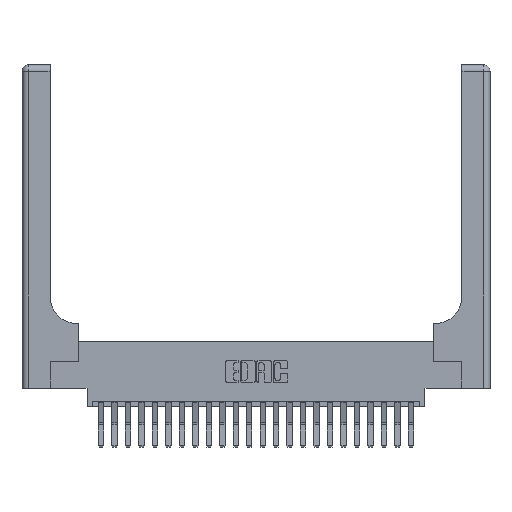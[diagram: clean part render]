
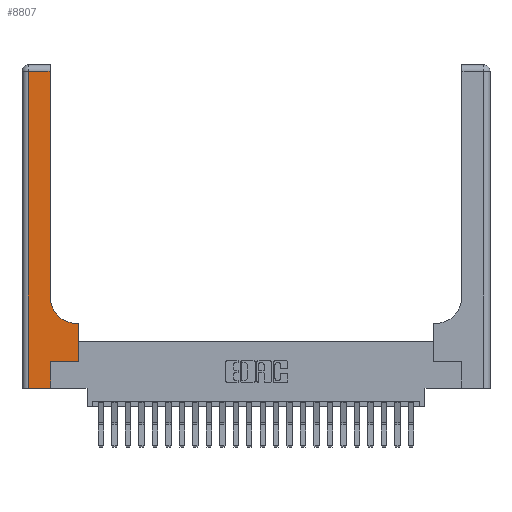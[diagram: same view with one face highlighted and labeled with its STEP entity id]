
A CAD part, top view. The second image highlights one B-rep face of the part: STEP entity #8807.
In plain terms, the highlighted planar face has unit normal (0, 0, 1).
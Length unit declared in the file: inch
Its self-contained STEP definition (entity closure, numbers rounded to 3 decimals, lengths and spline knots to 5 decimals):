
#568 = CARTESIAN_POINT ( 'NONE',  ( 0.265, 0., 0.37 ) ) ;
#609 = LINE ( 'NONE', #568, #10278 ) ;
#638 = CARTESIAN_POINT ( 'NONE',  ( 0.265, 0.25, 0.37 ) ) ;
#808 = ORIENTED_EDGE ( 'NONE', *, *, #5262, .T. ) ;
#1343 = CARTESIAN_POINT ( 'NONE',  ( 0.26, 0.6, 0.37 ) ) ;
#1937 = VERTEX_POINT ( 'NONE', #22433 ) ;
#2376 = ORIENTED_EDGE ( 'NONE', *, *, #13776, .T. ) ;
#2564 = AXIS2_PLACEMENT_3D ( 'NONE', #23322, #5184, #17915 ) ;
#2583 = DIRECTION ( 'NONE',  ( 0., 1., 0. ) ) ;
#2794 = CARTESIAN_POINT ( 'NONE',  ( 0.265, 0., 0.37 ) ) ;
#3011 = CARTESIAN_POINT ( 'NONE',  ( 0.26, 0.85, 0.37 ) ) ;
#3311 = FACE_OUTER_BOUND ( 'NONE', #10077, .T. ) ;
#4153 = EDGE_CURVE ( 'NONE', #20471, #22160, #22026, .T. ) ;
#4465 = VERTEX_POINT ( 'NONE', #6949 ) ;
#5184 = DIRECTION ( 'NONE',  ( 0., 0., -1. ) ) ;
#5262 = EDGE_CURVE ( 'NONE', #18649, #18373, #609, .T. ) ;
#5663 = LINE ( 'NONE', #18092, #20139 ) ;
#5691 = CARTESIAN_POINT ( 'NONE',  ( 0.51, 0.85, 0.37 ) ) ;
#5814 = EDGE_CURVE ( 'NONE', #19617, #18649, #13933, .T. ) ;
#6398 = ORIENTED_EDGE ( 'NONE', *, *, #19377, .T. ) ;
#6949 = CARTESIAN_POINT ( 'NONE',  ( 0.26, 2.94, 0.37 ) ) ;
#7015 = CARTESIAN_POINT ( 'NONE',  ( 0., 0., 0.37 ) ) ;
#7230 = ORIENTED_EDGE ( 'NONE', *, *, #4153, .T. ) ;
#7410 = CARTESIAN_POINT ( 'NONE',  ( 0.06, 0., 0.37 ) ) ;
#7495 = DIRECTION ( 'NONE',  ( 1., 0., 0. ) ) ;
#8097 = CARTESIAN_POINT ( 'NONE',  ( 0.528, 0.6, 0.37 ) ) ;
#8179 = VERTEX_POINT ( 'NONE', #3011 ) ;
#8243 = VECTOR ( 'NONE', #8671, 39.37008 ) ;
#8302 = EDGE_CURVE ( 'NONE', #21904, #8179, #17270, .T. ) ;
#8671 = DIRECTION ( 'NONE',  ( 0., -1., 0. ) ) ;
#8807 = ADVANCED_FACE ( 'NONE', ( #3311 ), #16079, .F. ) ;
#8955 = DIRECTION ( 'NONE',  ( 0., 1., 0. ) ) ;
#10077 = EDGE_LOOP ( 'NONE', ( #18849, #14893, #2376, #11867, #808, #22920, #7230, #6398, #19889 ) ) ;
#10278 = VECTOR ( 'NONE', #18729, 39.37008 ) ;
#10644 = DIRECTION ( 'NONE',  ( -1., 0., 0. ) ) ;
#10809 = AXIS2_PLACEMENT_3D ( 'NONE', #5691, #18401, #7495 ) ;
#11588 = CARTESIAN_POINT ( 'NONE',  ( 0.528, 0.25, 0.37 ) ) ;
#11867 = ORIENTED_EDGE ( 'NONE', *, *, #5814, .T. ) ;
#12570 = CARTESIAN_POINT ( 'NONE',  ( 0.51, 0.6, 0.37 ) ) ;
#13353 = DIRECTION ( 'NONE',  ( 1., 0., 0. ) ) ;
#13381 = VECTOR ( 'NONE', #17893, 39.37008 ) ;
#13773 = VECTOR ( 'NONE', #13353, 39.37008 ) ;
#13776 = EDGE_CURVE ( 'NONE', #1937, #19617, #17349, .T. ) ;
#13933 = LINE ( 'NONE', #7015, #13381 ) ;
#14123 = VECTOR ( 'NONE', #10644, 39.37008 ) ;
#14893 = ORIENTED_EDGE ( 'NONE', *, *, #16024, .T. ) ;
#15389 = CARTESIAN_POINT ( 'NONE',  ( 0.528, 0.25, 0.37 ) ) ;
#16024 = EDGE_CURVE ( 'NONE', #4465, #1937, #20056, .T. ) ;
#16079 = PLANE ( 'NONE',  #2564 ) ;
#16625 = CARTESIAN_POINT ( 'NONE',  ( 0.265, 0.25, 0.37 ) ) ;
#17228 = VECTOR ( 'NONE', #2583, 39.37008 ) ;
#17270 = CIRCLE ( 'NONE', #10809, 0.25 ) ;
#17349 = LINE ( 'NONE', #19541, #8243 ) ;
#17352 = EDGE_CURVE ( 'NONE', #18373, #20471, #22865, .T. ) ;
#17893 = DIRECTION ( 'NONE',  ( 1., 0., 0. ) ) ;
#17915 = DIRECTION ( 'NONE',  ( -1., 0., 0. ) ) ;
#18092 = CARTESIAN_POINT ( 'NONE',  ( 0.26, 3., 0.37 ) ) ;
#18373 = VERTEX_POINT ( 'NONE', #16625 ) ;
#18401 = DIRECTION ( 'NONE',  ( 0., 0., -1. ) ) ;
#18649 = VERTEX_POINT ( 'NONE', #2794 ) ;
#18729 = DIRECTION ( 'NONE',  ( 0., 1., 0. ) ) ;
#18849 = ORIENTED_EDGE ( 'NONE', *, *, #19521, .T. ) ;
#19377 = EDGE_CURVE ( 'NONE', #22160, #21904, #22444, .T. ) ;
#19426 = DIRECTION ( 'NONE',  ( -1., 0., 0. ) ) ;
#19521 = EDGE_CURVE ( 'NONE', #8179, #4465, #5663, .T. ) ;
#19541 = CARTESIAN_POINT ( 'NONE',  ( 0.06, 3., 0.37 ) ) ;
#19617 = VERTEX_POINT ( 'NONE', #7410 ) ;
#19889 = ORIENTED_EDGE ( 'NONE', *, *, #8302, .T. ) ;
#20056 = LINE ( 'NONE', #21489, #14123 ) ;
#20139 = VECTOR ( 'NONE', #8955, 39.37008 ) ;
#20471 = VERTEX_POINT ( 'NONE', #15389 ) ;
#21489 = CARTESIAN_POINT ( 'NONE',  ( 0., 2.94, 0.37 ) ) ;
#21904 = VERTEX_POINT ( 'NONE', #12570 ) ;
#22026 = LINE ( 'NONE', #11588, #17228 ) ;
#22160 = VERTEX_POINT ( 'NONE', #8097 ) ;
#22433 = CARTESIAN_POINT ( 'NONE',  ( 0.06, 2.94, 0.37 ) ) ;
#22444 = LINE ( 'NONE', #1343, #23026 ) ;
#22865 = LINE ( 'NONE', #638, #13773 ) ;
#22920 = ORIENTED_EDGE ( 'NONE', *, *, #17352, .T. ) ;
#23026 = VECTOR ( 'NONE', #19426, 39.37008 ) ;
#23322 = CARTESIAN_POINT ( 'NONE',  ( 0., 3., 0.37 ) ) ;
